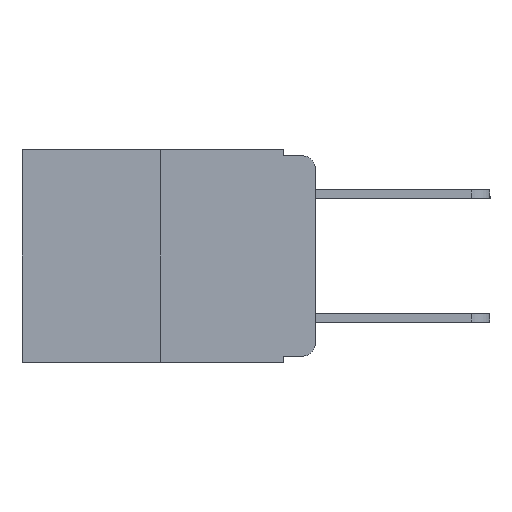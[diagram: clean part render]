
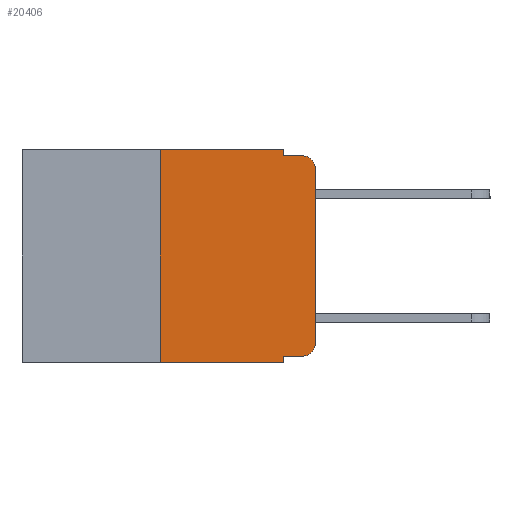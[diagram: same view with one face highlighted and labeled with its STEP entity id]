
A CAD part, left-side view. The second image highlights one B-rep face of the part: STEP entity #20406.
In plain terms, the highlighted planar face has unit normal (-1, 0, 0).
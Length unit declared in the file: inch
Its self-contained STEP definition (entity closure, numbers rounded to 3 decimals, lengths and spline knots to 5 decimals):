
#106 = CARTESIAN_POINT ( 'NONE',  ( 0., 0.02, -0.333 ) ) ;
#581 = VERTEX_POINT ( 'NONE', #13477 ) ;
#587 = VECTOR ( 'NONE', #3623, 39.37008 ) ;
#1263 = VECTOR ( 'NONE', #1425, 39.37008 ) ;
#1425 = DIRECTION ( 'NONE',  ( 0., -1., 0. ) ) ;
#1572 = EDGE_CURVE ( 'NONE', #24486, #13845, #6701, .T. ) ;
#1943 = ORIENTED_EDGE ( 'NONE', *, *, #24539, .T. ) ;
#2106 = CIRCLE ( 'NONE', #2572, 0.02 ) ;
#2147 = DIRECTION ( 'NONE',  ( 0., -1., 0. ) ) ;
#2195 = CARTESIAN_POINT ( 'NONE',  ( 0., 0.473, 0. ) ) ;
#2572 = AXIS2_PLACEMENT_3D ( 'NONE', #11765, #25465, #13730 ) ;
#2905 = CARTESIAN_POINT ( 'NONE',  ( 0., 0.473, 0. ) ) ;
#3016 = CARTESIAN_POINT ( 'NONE',  ( 0., 0.051, -0.333 ) ) ;
#3623 = DIRECTION ( 'NONE',  ( 0., -1., 0. ) ) ;
#4042 = LINE ( 'NONE', #4455, #24549 ) ;
#4455 = CARTESIAN_POINT ( 'NONE',  ( 0., 0.051, -0.333 ) ) ;
#5146 = DIRECTION ( 'NONE',  ( 0., 0., -1. ) ) ;
#5219 = CARTESIAN_POINT ( 'NONE',  ( 0., 0.051, -0.01 ) ) ;
#5462 = CARTESIAN_POINT ( 'NONE',  ( 0., 0.25, 0. ) ) ;
#5555 = CARTESIAN_POINT ( 'NONE',  ( 0., 0.473, -0.343 ) ) ;
#5595 = DIRECTION ( 'NONE',  ( -1., 0., 0. ) ) ;
#5792 = CARTESIAN_POINT ( 'NONE',  ( 0., 0.02, -0.01 ) ) ;
#6355 = VECTOR ( 'NONE', #9665, 39.37008 ) ;
#6512 = DIRECTION ( 'NONE',  ( 0., -1., 0. ) ) ;
#6701 = LINE ( 'NONE', #2905, #1263 ) ;
#6878 = VERTEX_POINT ( 'NONE', #5219 ) ;
#7679 = VERTEX_POINT ( 'NONE', #8038 ) ;
#8038 = CARTESIAN_POINT ( 'NONE',  ( 0., 0.051, -0.343 ) ) ;
#8252 = ORIENTED_EDGE ( 'NONE', *, *, #15182, .T. ) ;
#8320 = DIRECTION ( 'NONE',  ( 0., 0., -1. ) ) ;
#8621 = VECTOR ( 'NONE', #2147, 39.37008 ) ;
#9176 = VERTEX_POINT ( 'NONE', #5792 ) ;
#9625 = CARTESIAN_POINT ( 'NONE',  ( 0., 0.051, 0. ) ) ;
#9665 = DIRECTION ( 'NONE',  ( 0., 0., 1. ) ) ;
#9723 = CARTESIAN_POINT ( 'NONE',  ( 0., 0., 0. ) ) ;
#10350 = EDGE_CURVE ( 'NONE', #13304, #24486, #17603, .T. ) ;
#10871 = EDGE_CURVE ( 'NONE', #12741, #16064, #4042, .T. ) ;
#11221 = EDGE_CURVE ( 'NONE', #581, #9176, #22417, .T. ) ;
#11473 = CARTESIAN_POINT ( 'NONE',  ( 0., 0.051, 0. ) ) ;
#11583 = AXIS2_PLACEMENT_3D ( 'NONE', #17575, #5595, #19545 ) ;
#11765 = CARTESIAN_POINT ( 'NONE',  ( 0., 0.02, -0.313 ) ) ;
#12597 = FACE_OUTER_BOUND ( 'NONE', #19244, .T. ) ;
#12741 = VERTEX_POINT ( 'NONE', #3016 ) ;
#13017 = ORIENTED_EDGE ( 'NONE', *, *, #1572, .F. ) ;
#13062 = ORIENTED_EDGE ( 'NONE', *, *, #10871, .T. ) ;
#13304 = VERTEX_POINT ( 'NONE', #20789 ) ;
#13443 = DIRECTION ( 'NONE',  ( 0., 0., -1. ) ) ;
#13477 = CARTESIAN_POINT ( 'NONE',  ( 0., 0., -0.03 ) ) ;
#13538 = VECTOR ( 'NONE', #13443, 39.37008 ) ;
#13730 = DIRECTION ( 'NONE',  ( 0., 0., -1. ) ) ;
#13845 = VERTEX_POINT ( 'NONE', #9625 ) ;
#15182 = EDGE_CURVE ( 'NONE', #17124, #581, #23602, .T. ) ;
#15211 = AXIS2_PLACEMENT_3D ( 'NONE', #2195, #20223, #8320 ) ;
#15630 = DIRECTION ( 'NONE',  ( 0., 0., 1. ) ) ;
#15672 = EDGE_CURVE ( 'NONE', #13845, #6878, #15915, .T. ) ;
#15915 = LINE ( 'NONE', #24919, #25688 ) ;
#16064 = VERTEX_POINT ( 'NONE', #106 ) ;
#16733 = ORIENTED_EDGE ( 'NONE', *, *, #10350, .F. ) ;
#17124 = VERTEX_POINT ( 'NONE', #22271 ) ;
#17575 = CARTESIAN_POINT ( 'NONE',  ( 0., 0.02, -0.03 ) ) ;
#17603 = LINE ( 'NONE', #23444, #6355 ) ;
#17761 = VECTOR ( 'NONE', #15630, 39.37008 ) ;
#19244 = EDGE_LOOP ( 'NONE', ( #8252, #24617, #23723, #25551, #13017, #16733, #1943, #21633, #13062, #21345 ) ) ;
#19545 = DIRECTION ( 'NONE',  ( 0., 0., -1. ) ) ;
#20085 = CARTESIAN_POINT ( 'NONE',  ( 0., 0.051, -0.01 ) ) ;
#20107 = EDGE_CURVE ( 'NONE', #12741, #7679, #24555, .T. ) ;
#20223 = DIRECTION ( 'NONE',  ( 1., 0., 0. ) ) ;
#20406 = ADVANCED_FACE ( 'NONE', ( #12597 ), #22075, .F. ) ;
#20613 = EDGE_CURVE ( 'NONE', #16064, #17124, #2106, .T. ) ;
#20789 = CARTESIAN_POINT ( 'NONE',  ( 0., 0.25, -0.343 ) ) ;
#21345 = ORIENTED_EDGE ( 'NONE', *, *, #20613, .T. ) ;
#21633 = ORIENTED_EDGE ( 'NONE', *, *, #20107, .F. ) ;
#22075 = PLANE ( 'NONE',  #15211 ) ;
#22271 = CARTESIAN_POINT ( 'NONE',  ( 0., 0., -0.313 ) ) ;
#22417 = CIRCLE ( 'NONE', #11583, 0.02 ) ;
#22501 = LINE ( 'NONE', #5555, #587 ) ;
#23444 = CARTESIAN_POINT ( 'NONE',  ( 0., 0.25, 0. ) ) ;
#23527 = EDGE_CURVE ( 'NONE', #6878, #9176, #24353, .T. ) ;
#23602 = LINE ( 'NONE', #9723, #17761 ) ;
#23723 = ORIENTED_EDGE ( 'NONE', *, *, #23527, .F. ) ;
#24353 = LINE ( 'NONE', #20085, #8621 ) ;
#24486 = VERTEX_POINT ( 'NONE', #5462 ) ;
#24539 = EDGE_CURVE ( 'NONE', #13304, #7679, #22501, .T. ) ;
#24549 = VECTOR ( 'NONE', #6512, 39.37008 ) ;
#24555 = LINE ( 'NONE', #11473, #13538 ) ;
#24617 = ORIENTED_EDGE ( 'NONE', *, *, #11221, .T. ) ;
#24919 = CARTESIAN_POINT ( 'NONE',  ( 0., 0.051, 0. ) ) ;
#25465 = DIRECTION ( 'NONE',  ( -1., 0., 0. ) ) ;
#25551 = ORIENTED_EDGE ( 'NONE', *, *, #15672, .F. ) ;
#25688 = VECTOR ( 'NONE', #5146, 39.37008 ) ;
